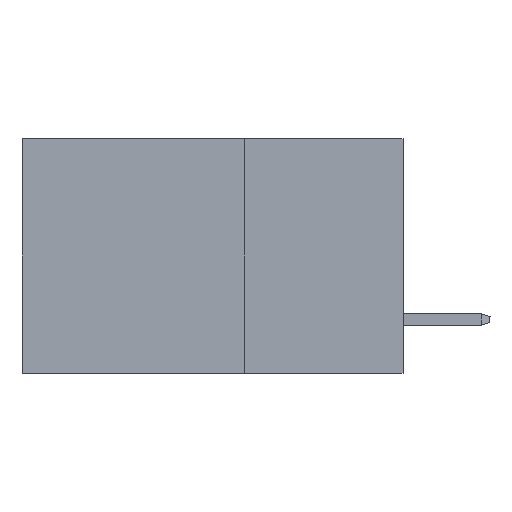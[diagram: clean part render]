
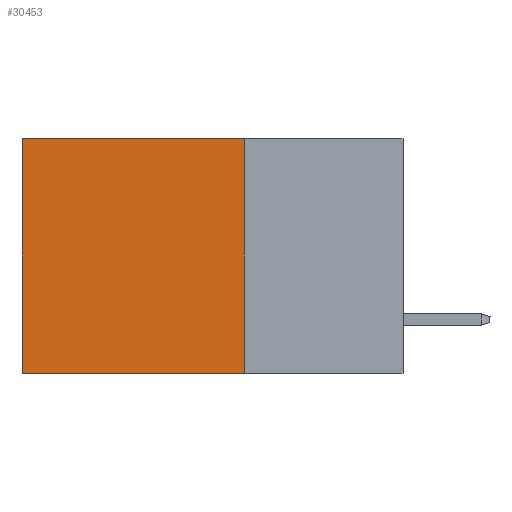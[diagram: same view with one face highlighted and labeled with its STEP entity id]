
A CAD part, left-side view. The second image highlights one B-rep face of the part: STEP entity #30453.
In plain terms, the highlighted planar face has unit normal (-1, 0, 0).
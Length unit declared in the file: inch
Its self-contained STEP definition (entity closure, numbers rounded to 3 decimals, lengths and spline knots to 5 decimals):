
#1946 = VERTEX_POINT ( 'NONE', #3051 ) ;
#2719 = ORIENTED_EDGE ( 'NONE', *, *, #39489, .F. ) ;
#3051 = CARTESIAN_POINT ( 'NONE',  ( 0.2875, 0.6, -0.37 ) ) ;
#5499 = DIRECTION ( 'NONE',  ( 0., 0., -1. ) ) ;
#5595 = ORIENTED_EDGE ( 'NONE', *, *, #35855, .T. ) ;
#5808 = DIRECTION ( 'NONE',  ( 0., 0., -1. ) ) ;
#6165 = CARTESIAN_POINT ( 'NONE',  ( 0.2875, 0.25, -0.37 ) ) ;
#7221 = VECTOR ( 'NONE', #28425, 39.37008 ) ;
#7288 = CARTESIAN_POINT ( 'NONE',  ( 0.2875, 0.6, 0. ) ) ;
#9241 = CARTESIAN_POINT ( 'NONE',  ( 0.2875, 0.25, 0. ) ) ;
#12530 = PLANE ( 'NONE',  #36112 ) ;
#13388 = CARTESIAN_POINT ( 'NONE',  ( 0.2875, 0.25, -0.37 ) ) ;
#15720 = CARTESIAN_POINT ( 'NONE',  ( 0.2875, 0.25, 0. ) ) ;
#17004 = VERTEX_POINT ( 'NONE', #39478 ) ;
#17992 = ORIENTED_EDGE ( 'NONE', *, *, #38168, .T. ) ;
#18714 = CARTESIAN_POINT ( 'NONE',  ( 0.2875, 0.25, 0. ) ) ;
#18853 = VERTEX_POINT ( 'NONE', #6165 ) ;
#21559 = LINE ( 'NONE', #21987, #40541 ) ;
#21639 = VECTOR ( 'NONE', #26399, 39.37008 ) ;
#21787 = LINE ( 'NONE', #9241, #7221 ) ;
#21898 = DIRECTION ( 'NONE',  ( 1., 0., 0. ) ) ;
#21987 = CARTESIAN_POINT ( 'NONE',  ( 0.2875, 0.6, 0. ) ) ;
#22280 = VECTOR ( 'NONE', #25341, 39.37008 ) ;
#25174 = EDGE_CURVE ( 'NONE', #17004, #18853, #21787, .T. ) ;
#25341 = DIRECTION ( 'NONE',  ( 0., 1., 0. ) ) ;
#25781 = FACE_OUTER_BOUND ( 'NONE', #34620, .T. ) ;
#26261 = ORIENTED_EDGE ( 'NONE', *, *, #25174, .F. ) ;
#26399 = DIRECTION ( 'NONE',  ( 0., 1., 0. ) ) ;
#28425 = DIRECTION ( 'NONE',  ( 0., 0., -1. ) ) ;
#29602 = LINE ( 'NONE', #13388, #21639 ) ;
#30453 = ADVANCED_FACE ( 'NONE', ( #25781 ), #12530, .F. ) ;
#34620 = EDGE_LOOP ( 'NONE', ( #5595, #2719, #26261, #17992 ) ) ;
#35770 = LINE ( 'NONE', #15720, #22280 ) ;
#35855 = EDGE_CURVE ( 'NONE', #38777, #1946, #21559, .T. ) ;
#36112 = AXIS2_PLACEMENT_3D ( 'NONE', #18714, #21898, #5499 ) ;
#38168 = EDGE_CURVE ( 'NONE', #17004, #38777, #35770, .T. ) ;
#38777 = VERTEX_POINT ( 'NONE', #7288 ) ;
#39478 = CARTESIAN_POINT ( 'NONE',  ( 0.2875, 0.25, 0. ) ) ;
#39489 = EDGE_CURVE ( 'NONE', #18853, #1946, #29602, .T. ) ;
#40541 = VECTOR ( 'NONE', #5808, 39.37008 ) ;
